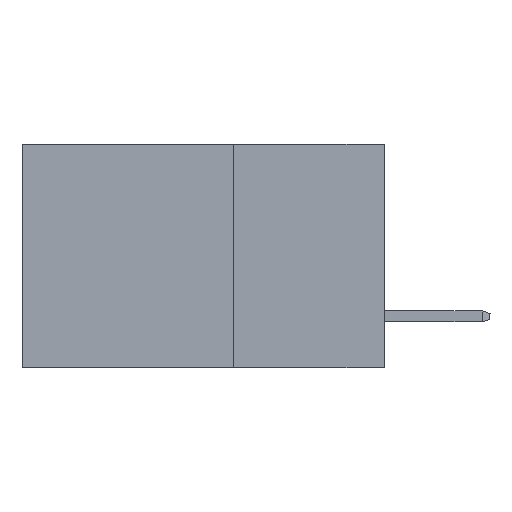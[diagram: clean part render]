
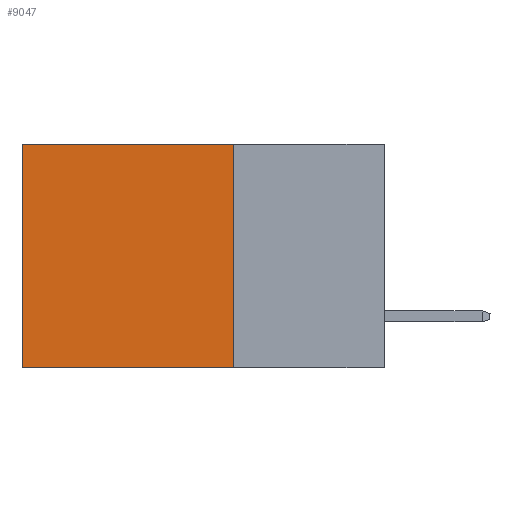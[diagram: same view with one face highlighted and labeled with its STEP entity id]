
A CAD part, left-side view. The second image highlights one B-rep face of the part: STEP entity #9047.
In plain terms, the highlighted planar face has unit normal (-1, 0, 0).
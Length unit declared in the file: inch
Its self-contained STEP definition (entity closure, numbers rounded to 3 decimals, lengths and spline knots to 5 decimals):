
#875 = DIRECTION ( 'NONE',  ( 0., 1., 0. ) ) ;
#1080 = DIRECTION ( 'NONE',  ( 0., 1., 0. ) ) ;
#1264 = VECTOR ( 'NONE', #15606, 39.37008 ) ;
#1585 = CARTESIAN_POINT ( 'NONE',  ( 0.2615, 0.25, -0.37 ) ) ;
#2378 = VERTEX_POINT ( 'NONE', #14557 ) ;
#2627 = CARTESIAN_POINT ( 'NONE',  ( 0.2615, 0.25, 0. ) ) ;
#2987 = ORIENTED_EDGE ( 'NONE', *, *, #6414, .F. ) ;
#5271 = EDGE_LOOP ( 'NONE', ( #9960, #16022, #2987, #10475 ) ) ;
#5293 = VERTEX_POINT ( 'NONE', #19188 ) ;
#6322 = CARTESIAN_POINT ( 'NONE',  ( 0.2615, 0.6, -0.37 ) ) ;
#6348 = DIRECTION ( 'NONE',  ( 0., 0., -1. ) ) ;
#6414 = EDGE_CURVE ( 'NONE', #13113, #5293, #11026, .T. ) ;
#7662 = FACE_OUTER_BOUND ( 'NONE', #5271, .T. ) ;
#7734 = EDGE_CURVE ( 'NONE', #8645, #2378, #8980, .T. ) ;
#8004 = DIRECTION ( 'NONE',  ( 0., 0., -1. ) ) ;
#8207 = VECTOR ( 'NONE', #1080, 39.37008 ) ;
#8471 = VECTOR ( 'NONE', #8004, 39.37008 ) ;
#8645 = VERTEX_POINT ( 'NONE', #18580 ) ;
#8980 = LINE ( 'NONE', #6322, #1264 ) ;
#9047 = ADVANCED_FACE ( 'NONE', ( #7662 ), #15143, .F. ) ;
#9960 = ORIENTED_EDGE ( 'NONE', *, *, #7734, .T. ) ;
#10475 = ORIENTED_EDGE ( 'NONE', *, *, #13648, .T. ) ;
#11026 = LINE ( 'NONE', #18893, #8471 ) ;
#11601 = EDGE_CURVE ( 'NONE', #5293, #2378, #13021, .T. ) ;
#13021 = LINE ( 'NONE', #19271, #17820 ) ;
#13113 = VERTEX_POINT ( 'NONE', #2627 ) ;
#13648 = EDGE_CURVE ( 'NONE', #13113, #8645, #19941, .T. ) ;
#14557 = CARTESIAN_POINT ( 'NONE',  ( 0.2615, 0.6, -0.37 ) ) ;
#15143 = PLANE ( 'NONE',  #15814 ) ;
#15238 = DIRECTION ( 'NONE',  ( 1., 0., 0. ) ) ;
#15606 = DIRECTION ( 'NONE',  ( 0., 0., -1. ) ) ;
#15814 = AXIS2_PLACEMENT_3D ( 'NONE', #1585, #15238, #6348 ) ;
#16022 = ORIENTED_EDGE ( 'NONE', *, *, #11601, .F. ) ;
#16895 = CARTESIAN_POINT ( 'NONE',  ( 0.2615, 0.25, 0. ) ) ;
#17820 = VECTOR ( 'NONE', #875, 39.37008 ) ;
#18580 = CARTESIAN_POINT ( 'NONE',  ( 0.2615, 0.6, 0. ) ) ;
#18893 = CARTESIAN_POINT ( 'NONE',  ( 0.2615, 0.25, -0.37 ) ) ;
#19188 = CARTESIAN_POINT ( 'NONE',  ( 0.2615, 0.25, -0.37 ) ) ;
#19271 = CARTESIAN_POINT ( 'NONE',  ( 0.2615, 0.25, -0.37 ) ) ;
#19941 = LINE ( 'NONE', #16895, #8207 ) ;
